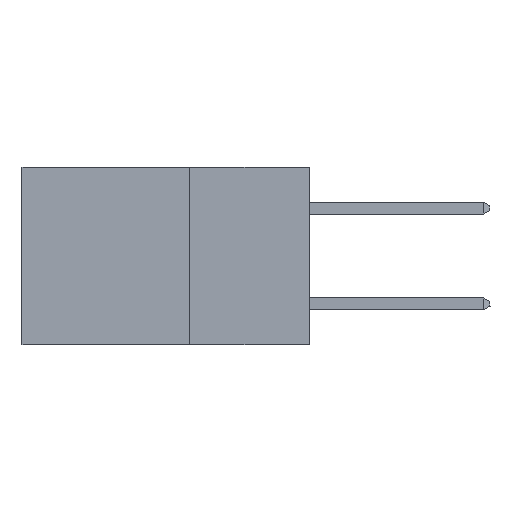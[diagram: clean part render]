
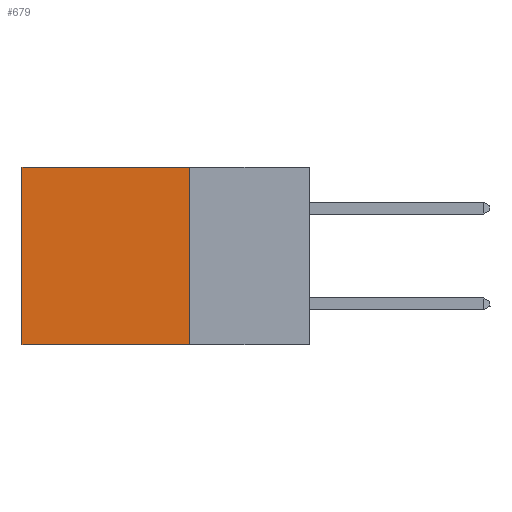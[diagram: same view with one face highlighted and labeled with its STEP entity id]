
A CAD part, left-side view. The second image highlights one B-rep face of the part: STEP entity #679.
In plain terms, the highlighted planar face has unit normal (-1, 0, 0).
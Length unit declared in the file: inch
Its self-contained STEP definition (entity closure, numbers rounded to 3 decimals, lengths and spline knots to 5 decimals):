
#224 = CARTESIAN_POINT ( 'NONE',  ( 0.2875, 0.25, 0. ) ) ;
#679 = ADVANCED_FACE ( 'NONE', ( #4428 ), #13934, .F. ) ;
#1247 = CARTESIAN_POINT ( 'NONE',  ( 0.2875, 0.25, -0.37 ) ) ;
#1386 = ORIENTED_EDGE ( 'NONE', *, *, #18154, .F. ) ;
#1648 = VECTOR ( 'NONE', #8821, 39.37008 ) ;
#2208 = EDGE_CURVE ( 'NONE', #11854, #18025, #8207, .T. ) ;
#2454 = ORIENTED_EDGE ( 'NONE', *, *, #13719, .T. ) ;
#3248 = DIRECTION ( 'NONE',  ( 0., 0., -1. ) ) ;
#3821 = EDGE_CURVE ( 'NONE', #11854, #14458, #13491, .T. ) ;
#4428 = FACE_OUTER_BOUND ( 'NONE', #17022, .T. ) ;
#4451 = CARTESIAN_POINT ( 'NONE',  ( 0.2875, 0.6, -0.37 ) ) ;
#4673 = CARTESIAN_POINT ( 'NONE',  ( 0.2875, 0.25, -0.37 ) ) ;
#5662 = VECTOR ( 'NONE', #3248, 39.37008 ) ;
#5729 = LINE ( 'NONE', #1247, #1648 ) ;
#8207 = LINE ( 'NONE', #8309, #11531 ) ;
#8309 = CARTESIAN_POINT ( 'NONE',  ( 0.2875, 0.25, 0. ) ) ;
#8355 = ORIENTED_EDGE ( 'NONE', *, *, #3821, .F. ) ;
#8821 = DIRECTION ( 'NONE',  ( 0., 1., 0. ) ) ;
#11025 = LINE ( 'NONE', #17523, #18441 ) ;
#11128 = DIRECTION ( 'NONE',  ( 0., 0., -1. ) ) ;
#11531 = VECTOR ( 'NONE', #16038, 39.37008 ) ;
#11854 = VERTEX_POINT ( 'NONE', #16945 ) ;
#12429 = DIRECTION ( 'NONE',  ( 1., 0., 0. ) ) ;
#12843 = ORIENTED_EDGE ( 'NONE', *, *, #2208, .T. ) ;
#12945 = CARTESIAN_POINT ( 'NONE',  ( 0.2875, 0.6, 0. ) ) ;
#13491 = LINE ( 'NONE', #18662, #5662 ) ;
#13719 = EDGE_CURVE ( 'NONE', #18025, #17857, #11025, .T. ) ;
#13934 = PLANE ( 'NONE',  #18978 ) ;
#14458 = VERTEX_POINT ( 'NONE', #4673 ) ;
#16038 = DIRECTION ( 'NONE',  ( 0., 1., 0. ) ) ;
#16945 = CARTESIAN_POINT ( 'NONE',  ( 0.2875, 0.25, 0. ) ) ;
#17022 = EDGE_LOOP ( 'NONE', ( #2454, #1386, #8355, #12843 ) ) ;
#17523 = CARTESIAN_POINT ( 'NONE',  ( 0.2875, 0.6, 0. ) ) ;
#17857 = VERTEX_POINT ( 'NONE', #4451 ) ;
#18025 = VERTEX_POINT ( 'NONE', #12945 ) ;
#18154 = EDGE_CURVE ( 'NONE', #14458, #17857, #5729, .T. ) ;
#18441 = VECTOR ( 'NONE', #11128, 39.37008 ) ;
#18540 = DIRECTION ( 'NONE',  ( 0., 0., -1. ) ) ;
#18662 = CARTESIAN_POINT ( 'NONE',  ( 0.2875, 0.25, 0. ) ) ;
#18978 = AXIS2_PLACEMENT_3D ( 'NONE', #224, #12429, #18540 ) ;
